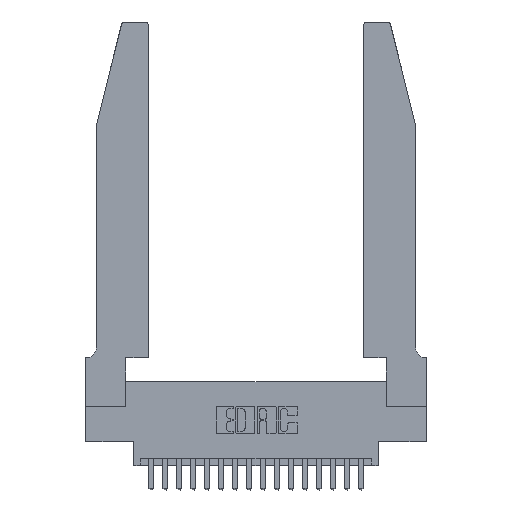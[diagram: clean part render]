
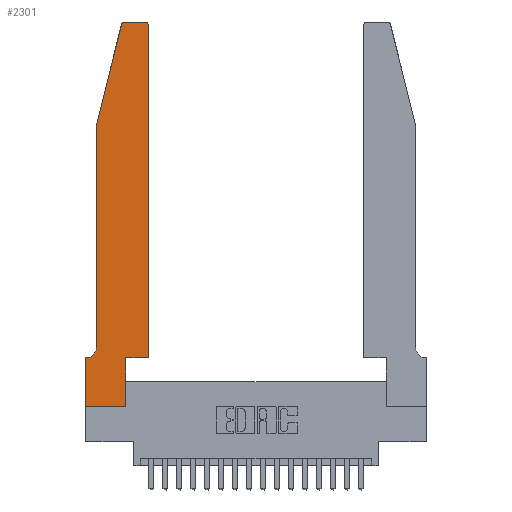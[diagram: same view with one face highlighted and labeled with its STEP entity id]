
A CAD part, top view. The second image highlights one B-rep face of the part: STEP entity #2301.
In plain terms, the highlighted planar face has unit normal (0, 0, 1).
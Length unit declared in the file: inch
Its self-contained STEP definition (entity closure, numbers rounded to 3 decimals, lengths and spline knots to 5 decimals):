
#67 = VECTOR ( 'NONE', #20100, 39.37008 ) ;
#423 = ORIENTED_EDGE ( 'NONE', *, *, #1914, .T. ) ;
#496 = DIRECTION ( 'NONE',  ( 1., 0., 0. ) ) ;
#914 = VERTEX_POINT ( 'NONE', #4629 ) ;
#1462 = LINE ( 'NONE', #7116, #4372 ) ;
#1870 = DIRECTION ( 'NONE',  ( 0., -1., 0. ) ) ;
#1914 = EDGE_CURVE ( 'NONE', #7526, #12261, #18248, .T. ) ;
#2261 = ORIENTED_EDGE ( 'NONE', *, *, #13601, .T. ) ;
#2301 = ADVANCED_FACE ( 'NONE', ( #7909 ), #14383, .T. ) ;
#2379 = VERTEX_POINT ( 'NONE', #10968 ) ;
#2459 = CARTESIAN_POINT ( 'NONE',  ( 0.284, 2.72, 0.37 ) ) ;
#3133 = DIRECTION ( 'NONE',  ( -1., 0., 0. ) ) ;
#3370 = CARTESIAN_POINT ( 'NONE',  ( 0.4505, 0.35, 0.37 ) ) ;
#3844 = VECTOR ( 'NONE', #14097, 39.37008 ) ;
#3977 = ORIENTED_EDGE ( 'NONE', *, *, #11322, .T. ) ;
#4012 = EDGE_CURVE ( 'NONE', #2379, #12551, #9363, .T. ) ;
#4159 = DIRECTION ( 'NONE',  ( 1., 0., 0. ) ) ;
#4215 = CARTESIAN_POINT ( 'NONE',  ( 0.25487, 2.72718, 0.37 ) ) ;
#4348 = LINE ( 'NONE', #17471, #3844 ) ;
#4372 = VECTOR ( 'NONE', #496, 39.37008 ) ;
#4460 = ORIENTED_EDGE ( 'NONE', *, *, #10902, .T. ) ;
#4475 = VECTOR ( 'NONE', #1870, 39.37008 ) ;
#4505 = ORIENTED_EDGE ( 'NONE', *, *, #10159, .T. ) ;
#4629 = CARTESIAN_POINT ( 'NONE',  ( 0.284, 2.75, 0.37 ) ) ;
#4885 = EDGE_CURVE ( 'NONE', #8293, #16920, #18894, .T. ) ;
#5086 = DIRECTION ( 'NONE',  ( 0., 0., 1. ) ) ;
#5700 = CARTESIAN_POINT ( 'NONE',  ( 0.0055, 0.42, 0.37 ) ) ;
#6395 = CARTESIAN_POINT ( 'NONE',  ( 0.4205, 2.75, 0.37 ) ) ;
#6460 = CARTESIAN_POINT ( 'NONE',  ( 0.0055, 0.35, 0.37 ) ) ;
#6481 = CARTESIAN_POINT ( 'NONE',  ( 0.2865, 0.35, 0.37 ) ) ;
#6859 = CARTESIAN_POINT ( 'NONE',  ( 0.0755, 2., 0.37 ) ) ;
#7066 = ORIENTED_EDGE ( 'NONE', *, *, #10072, .T. ) ;
#7116 = CARTESIAN_POINT ( 'NONE',  ( 0.4505, 0.35, 0.37 ) ) ;
#7319 = DIRECTION ( 'NONE',  ( -1., 0., 0. ) ) ;
#7401 = ORIENTED_EDGE ( 'NONE', *, *, #16773, .T. ) ;
#7526 = VERTEX_POINT ( 'NONE', #14160 ) ;
#7909 = FACE_OUTER_BOUND ( 'NONE', #16158, .T. ) ;
#8283 = AXIS2_PLACEMENT_3D ( 'NONE', #5700, #16949, #7319 ) ;
#8293 = VERTEX_POINT ( 'NONE', #6460 ) ;
#8699 = AXIS2_PLACEMENT_3D ( 'NONE', #14464, #14339, #14272 ) ;
#8841 = VERTEX_POINT ( 'NONE', #14234 ) ;
#9363 = LINE ( 'NONE', #10441, #67 ) ;
#9488 = ORIENTED_EDGE ( 'NONE', *, *, #4012, .T. ) ;
#9495 = CIRCLE ( 'NONE', #14119, 0.03 ) ;
#9657 = VECTOR ( 'NONE', #10756, 39.37008 ) ;
#9781 = CARTESIAN_POINT ( 'NONE',  ( 0., 0.35, 0.37 ) ) ;
#9990 = CARTESIAN_POINT ( 'NONE',  ( 0., 0., 0.37 ) ) ;
#10022 = CIRCLE ( 'NONE', #16931, 0.03 ) ;
#10072 = EDGE_CURVE ( 'NONE', #8841, #12759, #10248, .T. ) ;
#10159 = EDGE_CURVE ( 'NONE', #16920, #13882, #13003, .T. ) ;
#10248 = LINE ( 'NONE', #3370, #14502 ) ;
#10368 = EDGE_CURVE ( 'NONE', #914, #15879, #9495, .T. ) ;
#10441 = CARTESIAN_POINT ( 'NONE',  ( 0.0755, 2., 0.37 ) ) ;
#10756 = DIRECTION ( 'NONE',  ( 0., 1., 0. ) ) ;
#10902 = EDGE_CURVE ( 'NONE', #12551, #8293, #12208, .T. ) ;
#10968 = CARTESIAN_POINT ( 'NONE',  ( 0.0755, 2., 0.37 ) ) ;
#11322 = EDGE_CURVE ( 'NONE', #15879, #2379, #20285, .T. ) ;
#11599 = CARTESIAN_POINT ( 'NONE',  ( 0., 0., 0.37 ) ) ;
#11644 = DIRECTION ( 'NONE',  ( 1., 0., 0. ) ) ;
#11670 = DIRECTION ( 'NONE',  ( -0.239, -0.971, 0. ) ) ;
#12029 = ORIENTED_EDGE ( 'NONE', *, *, #10368, .T. ) ;
#12208 = CIRCLE ( 'NONE', #8283, 0.07 ) ;
#12261 = VERTEX_POINT ( 'NONE', #6481 ) ;
#12263 = ORIENTED_EDGE ( 'NONE', *, *, #4885, .T. ) ;
#12455 = CARTESIAN_POINT ( 'NONE',  ( 0.4505, 2.72, 0.37 ) ) ;
#12551 = VERTEX_POINT ( 'NONE', #15206 ) ;
#12759 = VERTEX_POINT ( 'NONE', #12455 ) ;
#13003 = LINE ( 'NONE', #11599, #4475 ) ;
#13274 = CARTESIAN_POINT ( 'NONE',  ( 0., 0., 0.37 ) ) ;
#13554 = VECTOR ( 'NONE', #3133, 39.37008 ) ;
#13601 = EDGE_CURVE ( 'NONE', #12759, #17389, #10022, .T. ) ;
#13755 = DIRECTION ( 'NONE',  ( 0., 0., 1. ) ) ;
#13882 = VERTEX_POINT ( 'NONE', #13274 ) ;
#14097 = DIRECTION ( 'NONE',  ( -1., 0., 0. ) ) ;
#14119 = AXIS2_PLACEMENT_3D ( 'NONE', #2459, #13755, #4159 ) ;
#14160 = CARTESIAN_POINT ( 'NONE',  ( 0.2865, 0., 0.37 ) ) ;
#14234 = CARTESIAN_POINT ( 'NONE',  ( 0.4505, 0.35, 0.37 ) ) ;
#14272 = DIRECTION ( 'NONE',  ( 1., 0., 0. ) ) ;
#14339 = DIRECTION ( 'NONE',  ( 0., 0., 1. ) ) ;
#14383 = PLANE ( 'NONE',  #8699 ) ;
#14390 = CARTESIAN_POINT ( 'NONE',  ( 0.0755, 0.35, 0.37 ) ) ;
#14464 = CARTESIAN_POINT ( 'NONE',  ( 0., 0.35, 0.37 ) ) ;
#14502 = VECTOR ( 'NONE', #21056, 39.37008 ) ;
#14664 = CARTESIAN_POINT ( 'NONE',  ( 0.4205, 2.72, 0.37 ) ) ;
#14918 = VECTOR ( 'NONE', #11644, 39.37008 ) ;
#15206 = CARTESIAN_POINT ( 'NONE',  ( 0.0755, 0.42, 0.37 ) ) ;
#15879 = VERTEX_POINT ( 'NONE', #4215 ) ;
#15967 = VECTOR ( 'NONE', #11670, 39.37008 ) ;
#16158 = EDGE_LOOP ( 'NONE', ( #7401, #12029, #3977, #9488, #4460, #12263, #4505, #18399, #423, #18664, #7066, #2261 ) ) ;
#16324 = DIRECTION ( 'NONE',  ( 1., 0., 0. ) ) ;
#16488 = CARTESIAN_POINT ( 'NONE',  ( 0.2865, 0.35, 0.37 ) ) ;
#16773 = EDGE_CURVE ( 'NONE', #17389, #914, #4348, .T. ) ;
#16920 = VERTEX_POINT ( 'NONE', #9781 ) ;
#16931 = AXIS2_PLACEMENT_3D ( 'NONE', #14664, #5086, #16324 ) ;
#16949 = DIRECTION ( 'NONE',  ( 0., 0., -1. ) ) ;
#17389 = VERTEX_POINT ( 'NONE', #6395 ) ;
#17471 = CARTESIAN_POINT ( 'NONE',  ( 0.2605, 2.75, 0.37 ) ) ;
#17494 = LINE ( 'NONE', #9990, #14918 ) ;
#18248 = LINE ( 'NONE', #16488, #9657 ) ;
#18399 = ORIENTED_EDGE ( 'NONE', *, *, #20651, .T. ) ;
#18664 = ORIENTED_EDGE ( 'NONE', *, *, #20756, .T. ) ;
#18894 = LINE ( 'NONE', #14390, #13554 ) ;
#20100 = DIRECTION ( 'NONE',  ( 0., -1., 0. ) ) ;
#20285 = LINE ( 'NONE', #6859, #15967 ) ;
#20651 = EDGE_CURVE ( 'NONE', #13882, #7526, #17494, .T. ) ;
#20756 = EDGE_CURVE ( 'NONE', #12261, #8841, #1462, .T. ) ;
#21056 = DIRECTION ( 'NONE',  ( 0., 1., 0. ) ) ;
